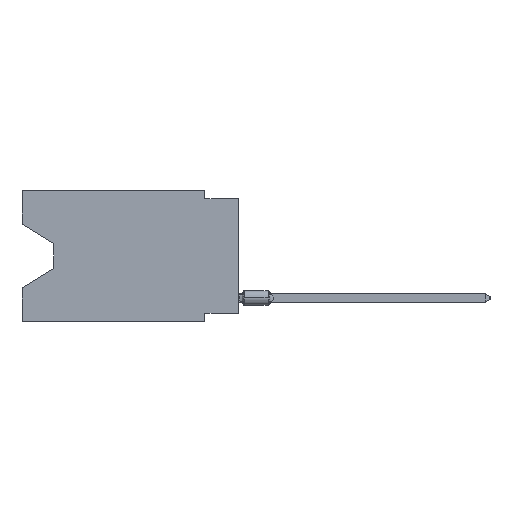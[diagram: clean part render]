
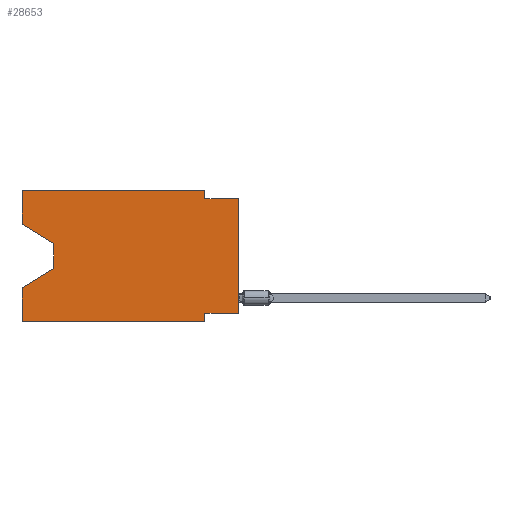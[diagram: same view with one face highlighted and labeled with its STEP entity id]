
A CAD part, left-side view. The second image highlights one B-rep face of the part: STEP entity #28653.
In plain terms, the highlighted planar face has unit normal (-1, 0, 0).
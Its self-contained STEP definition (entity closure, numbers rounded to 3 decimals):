
#358 = DIRECTION ( 'NONE',  ( 0., -1., 0. ) ) ;
#1549 = VECTOR ( 'NONE', #30061, 1000. ) ;
#1639 = DIRECTION ( 'NONE',  ( 1., 0., 0. ) ) ;
#1652 = CARTESIAN_POINT ( 'NONE',  ( 0., 0., -9.271 ) ) ;
#2006 = VERTEX_POINT ( 'NONE', #40015 ) ;
#2391 = CARTESIAN_POINT ( 'NONE',  ( 0., 13.97, -4.013 ) ) ;
#2422 = LINE ( 'NONE', #40712, #50338 ) ;
#2931 = ORIENTED_EDGE ( 'NONE', *, *, #39995, .F. ) ;
#3970 = VECTOR ( 'NONE', #8244, 1000. ) ;
#4417 = DIRECTION ( 'NONE',  ( 0., 0., -1. ) ) ;
#4510 = VERTEX_POINT ( 'NONE', #18513 ) ;
#4872 = CARTESIAN_POINT ( 'NONE',  ( 0., 2.54, -9.906 ) ) ;
#5496 = DIRECTION ( 'NONE',  ( 0., 0., 1. ) ) ;
#6213 = VERTEX_POINT ( 'NONE', #19358 ) ;
#6588 = VERTEX_POINT ( 'NONE', #4872 ) ;
#6644 = LINE ( 'NONE', #31425, #21891 ) ;
#7241 = VECTOR ( 'NONE', #8583, 1000. ) ;
#7403 = LINE ( 'NONE', #2391, #50284 ) ;
#7434 = DIRECTION ( 'NONE',  ( 0., 1., 0. ) ) ;
#7471 = ORIENTED_EDGE ( 'NONE', *, *, #13715, .T. ) ;
#7526 = ORIENTED_EDGE ( 'NONE', *, *, #45905, .T. ) ;
#8244 = DIRECTION ( 'NONE',  ( 0., 0., 1. ) ) ;
#8583 = DIRECTION ( 'NONE',  ( 0., -0.855, -0.519 ) ) ;
#8721 = DIRECTION ( 'NONE',  ( 0., 0., -1. ) ) ;
#9999 = CARTESIAN_POINT ( 'NONE',  ( 0., 2.54, 0. ) ) ;
#13207 = CARTESIAN_POINT ( 'NONE',  ( 0., 16.383, 0. ) ) ;
#13216 = CARTESIAN_POINT ( 'NONE',  ( 0., 2.54, -9.271 ) ) ;
#13715 = EDGE_CURVE ( 'NONE', #57311, #6588, #24205, .T. ) ;
#13781 = VECTOR ( 'NONE', #33245, 1000. ) ;
#15464 = VECTOR ( 'NONE', #358, 1000. ) ;
#17319 = ORIENTED_EDGE ( 'NONE', *, *, #18390, .F. ) ;
#17351 = CARTESIAN_POINT ( 'NONE',  ( 0., 16.383, 0. ) ) ;
#18390 = EDGE_CURVE ( 'NONE', #2006, #6213, #48624, .T. ) ;
#18513 = CARTESIAN_POINT ( 'NONE',  ( 0., 2.54, 0. ) ) ;
#19358 = CARTESIAN_POINT ( 'NONE',  ( 0., 0., -0.635 ) ) ;
#19599 = CARTESIAN_POINT ( 'NONE',  ( 0., 16.383, 0. ) ) ;
#19830 = PLANE ( 'NONE',  #50335 ) ;
#20126 = VERTEX_POINT ( 'NONE', #13216 ) ;
#21383 = LINE ( 'NONE', #37057, #49970 ) ;
#21891 = VECTOR ( 'NONE', #50586, 1000. ) ;
#22331 = CARTESIAN_POINT ( 'NONE',  ( 0., 13.97, -4.013 ) ) ;
#23543 = ORIENTED_EDGE ( 'NONE', *, *, #54216, .T. ) ;
#24205 = LINE ( 'NONE', #43370, #15464 ) ;
#24713 = CARTESIAN_POINT ( 'NONE',  ( 0., 13.97, -5.893 ) ) ;
#25066 = CARTESIAN_POINT ( 'NONE',  ( 0., 0., -0.635 ) ) ;
#25493 = FACE_OUTER_BOUND ( 'NONE', #50085, .T. ) ;
#26410 = EDGE_CURVE ( 'NONE', #48599, #20126, #2422, .T. ) ;
#27353 = ORIENTED_EDGE ( 'NONE', *, *, #27874, .F. ) ;
#27874 = EDGE_CURVE ( 'NONE', #20126, #6588, #48045, .T. ) ;
#28653 = ADVANCED_FACE ( 'NONE', ( #25493 ), #19830, .F. ) ;
#29865 = CARTESIAN_POINT ( 'NONE',  ( 0., 16.383, -7.36 ) ) ;
#29975 = LINE ( 'NONE', #19599, #56640 ) ;
#30008 = EDGE_CURVE ( 'NONE', #61457, #56567, #29975, .T. ) ;
#30061 = DIRECTION ( 'NONE',  ( 0., 0.855, -0.519 ) ) ;
#30631 = CARTESIAN_POINT ( 'NONE',  ( 0., 16.383, -9.906 ) ) ;
#31425 = CARTESIAN_POINT ( 'NONE',  ( 0., 16.383, 0. ) ) ;
#31634 = ORIENTED_EDGE ( 'NONE', *, *, #59022, .F. ) ;
#33245 = DIRECTION ( 'NONE',  ( 0., 0., -1. ) ) ;
#34454 = LINE ( 'NONE', #24713, #1549 ) ;
#34594 = CARTESIAN_POINT ( 'NONE',  ( 0., 13.97, -5.893 ) ) ;
#35628 = ORIENTED_EDGE ( 'NONE', *, *, #42749, .F. ) ;
#36631 = VERTEX_POINT ( 'NONE', #29865 ) ;
#37057 = CARTESIAN_POINT ( 'NONE',  ( 0., 0., 0. ) ) ;
#37769 = CARTESIAN_POINT ( 'NONE',  ( 0., 16.383, -2.546 ) ) ;
#39056 = ORIENTED_EDGE ( 'NONE', *, *, #39109, .T. ) ;
#39109 = EDGE_CURVE ( 'NONE', #56593, #41190, #7403, .T. ) ;
#39995 = EDGE_CURVE ( 'NONE', #56567, #4510, #6644, .T. ) ;
#40015 = CARTESIAN_POINT ( 'NONE',  ( 0., 2.54, -0.635 ) ) ;
#40068 = EDGE_CURVE ( 'NONE', #48599, #6213, #21383, .T. ) ;
#40712 = CARTESIAN_POINT ( 'NONE',  ( 0., 0., -9.271 ) ) ;
#41190 = VERTEX_POINT ( 'NONE', #34594 ) ;
#41833 = LINE ( 'NONE', #17351, #3970 ) ;
#42749 = EDGE_CURVE ( 'NONE', #57311, #36631, #41833, .T. ) ;
#42974 = LINE ( 'NONE', #9999, #13781 ) ;
#43329 = CARTESIAN_POINT ( 'NONE',  ( 0., 2.54, -9.906 ) ) ;
#43370 = CARTESIAN_POINT ( 'NONE',  ( 0., 16.383, -9.906 ) ) ;
#43409 = VECTOR ( 'NONE', #4417, 1000. ) ;
#44227 = DIRECTION ( 'NONE',  ( 0., -1., 0. ) ) ;
#44643 = CARTESIAN_POINT ( 'NONE',  ( 0., 16.383, 0. ) ) ;
#45905 = EDGE_CURVE ( 'NONE', #61457, #56593, #51622, .T. ) ;
#45940 = ORIENTED_EDGE ( 'NONE', *, *, #26410, .F. ) ;
#46631 = DIRECTION ( 'NONE',  ( 0., 0., -1. ) ) ;
#46991 = VECTOR ( 'NONE', #44227, 1000. ) ;
#48045 = LINE ( 'NONE', #43329, #43409 ) ;
#48599 = VERTEX_POINT ( 'NONE', #1652 ) ;
#48624 = LINE ( 'NONE', #25066, #46991 ) ;
#49970 = VECTOR ( 'NONE', #56234, 1000. ) ;
#50085 = EDGE_LOOP ( 'NONE', ( #7526, #39056, #23543, #35628, #7471, #27353, #45940, #62109, #17319, #31634, #2931, #58831 ) ) ;
#50284 = VECTOR ( 'NONE', #46631, 1000. ) ;
#50335 = AXIS2_PLACEMENT_3D ( 'NONE', #44643, #1639, #8721 ) ;
#50338 = VECTOR ( 'NONE', #7434, 1000. ) ;
#50586 = DIRECTION ( 'NONE',  ( 0., -1., 0. ) ) ;
#51622 = LINE ( 'NONE', #37769, #7241 ) ;
#54216 = EDGE_CURVE ( 'NONE', #41190, #36631, #34454, .T. ) ;
#56234 = DIRECTION ( 'NONE',  ( 0., 0., 1. ) ) ;
#56567 = VERTEX_POINT ( 'NONE', #13207 ) ;
#56593 = VERTEX_POINT ( 'NONE', #22331 ) ;
#56630 = CARTESIAN_POINT ( 'NONE',  ( 0., 16.383, -2.546 ) ) ;
#56640 = VECTOR ( 'NONE', #5496, 1000. ) ;
#57311 = VERTEX_POINT ( 'NONE', #30631 ) ;
#58831 = ORIENTED_EDGE ( 'NONE', *, *, #30008, .F. ) ;
#59022 = EDGE_CURVE ( 'NONE', #4510, #2006, #42974, .T. ) ;
#61457 = VERTEX_POINT ( 'NONE', #56630 ) ;
#62109 = ORIENTED_EDGE ( 'NONE', *, *, #40068, .T. ) ;
